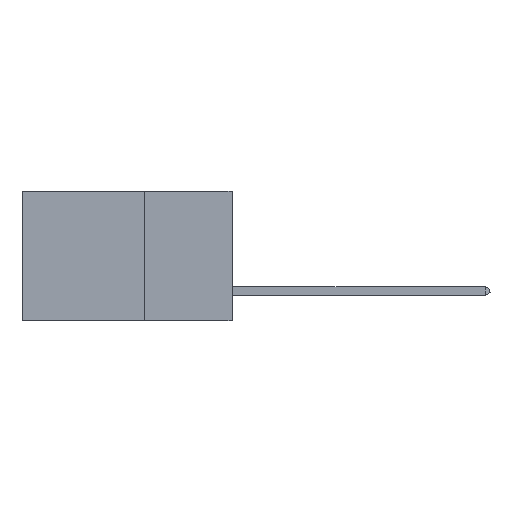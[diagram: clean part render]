
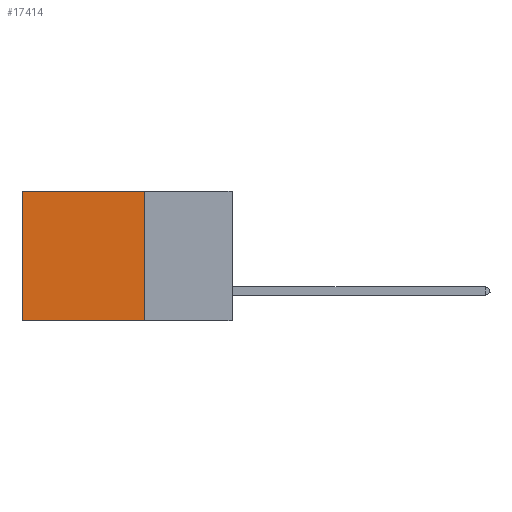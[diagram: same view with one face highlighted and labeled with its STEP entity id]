
A CAD part, left-side view. The second image highlights one B-rep face of the part: STEP entity #17414.
In plain terms, the highlighted planar face has unit normal (-1, 0, 0).
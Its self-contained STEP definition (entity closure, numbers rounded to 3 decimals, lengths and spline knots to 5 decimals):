
#8 = EDGE_CURVE ( 'NONE', #39199, #33204, #44453, .T. ) ;
#540 = CARTESIAN_POINT ( 'NONE',  ( 0.2875, 0.25, 0. ) ) ;
#1458 = ORIENTED_EDGE ( 'NONE', *, *, #7330, .T. ) ;
#2658 = VERTEX_POINT ( 'NONE', #30213 ) ;
#3255 = ORIENTED_EDGE ( 'NONE', *, *, #8, .F. ) ;
#5378 = EDGE_CURVE ( 'NONE', #33204, #2658, #47753, .T. ) ;
#6403 = CARTESIAN_POINT ( 'NONE',  ( 0.2875, 0.6, 0. ) ) ;
#7330 = EDGE_CURVE ( 'NONE', #39199, #30140, #37862, .T. ) ;
#7622 = DIRECTION ( 'NONE',  ( 0., 0., -1. ) ) ;
#9657 = CARTESIAN_POINT ( 'NONE',  ( 0.2875, 0.25, 0. ) ) ;
#9967 = CARTESIAN_POINT ( 'NONE',  ( 0.2875, 0.25, -0.37 ) ) ;
#12993 = EDGE_CURVE ( 'NONE', #30140, #2658, #36590, .T. ) ;
#17414 = ADVANCED_FACE ( 'NONE', ( #21844 ), #36818, .F. ) ;
#17921 = CARTESIAN_POINT ( 'NONE',  ( 0.2875, 0.25, -0.37 ) ) ;
#20472 = VECTOR ( 'NONE', #23113, 39.37008 ) ;
#21844 = FACE_OUTER_BOUND ( 'NONE', #33455, .T. ) ;
#23113 = DIRECTION ( 'NONE',  ( 0., 1., 0. ) ) ;
#25532 = CARTESIAN_POINT ( 'NONE',  ( 0.2875, 0.25, 0. ) ) ;
#29086 = DIRECTION ( 'NONE',  ( 0., 1., 0. ) ) ;
#29998 = VECTOR ( 'NONE', #7622, 39.37008 ) ;
#30140 = VERTEX_POINT ( 'NONE', #35832 ) ;
#30213 = CARTESIAN_POINT ( 'NONE',  ( 0.2875, 0.6, -0.37 ) ) ;
#30345 = VECTOR ( 'NONE', #29086, 39.37008 ) ;
#31231 = AXIS2_PLACEMENT_3D ( 'NONE', #25532, #46501, #46752 ) ;
#33204 = VERTEX_POINT ( 'NONE', #17921 ) ;
#33455 = EDGE_LOOP ( 'NONE', ( #39154, #33503, #3255, #1458 ) ) ;
#33503 = ORIENTED_EDGE ( 'NONE', *, *, #5378, .F. ) ;
#35832 = CARTESIAN_POINT ( 'NONE',  ( 0.2875, 0.6, 0. ) ) ;
#36590 = LINE ( 'NONE', #6403, #48165 ) ;
#36818 = PLANE ( 'NONE',  #31231 ) ;
#37862 = LINE ( 'NONE', #540, #20472 ) ;
#39154 = ORIENTED_EDGE ( 'NONE', *, *, #12993, .T. ) ;
#39199 = VERTEX_POINT ( 'NONE', #9657 ) ;
#44453 = LINE ( 'NONE', #44692, #29998 ) ;
#44455 = DIRECTION ( 'NONE',  ( 0., 0., -1. ) ) ;
#44692 = CARTESIAN_POINT ( 'NONE',  ( 0.2875, 0.25, 0. ) ) ;
#46501 = DIRECTION ( 'NONE',  ( 1., 0., 0. ) ) ;
#46752 = DIRECTION ( 'NONE',  ( 0., 0., -1. ) ) ;
#47753 = LINE ( 'NONE', #9967, #30345 ) ;
#48165 = VECTOR ( 'NONE', #44455, 39.37008 ) ;
